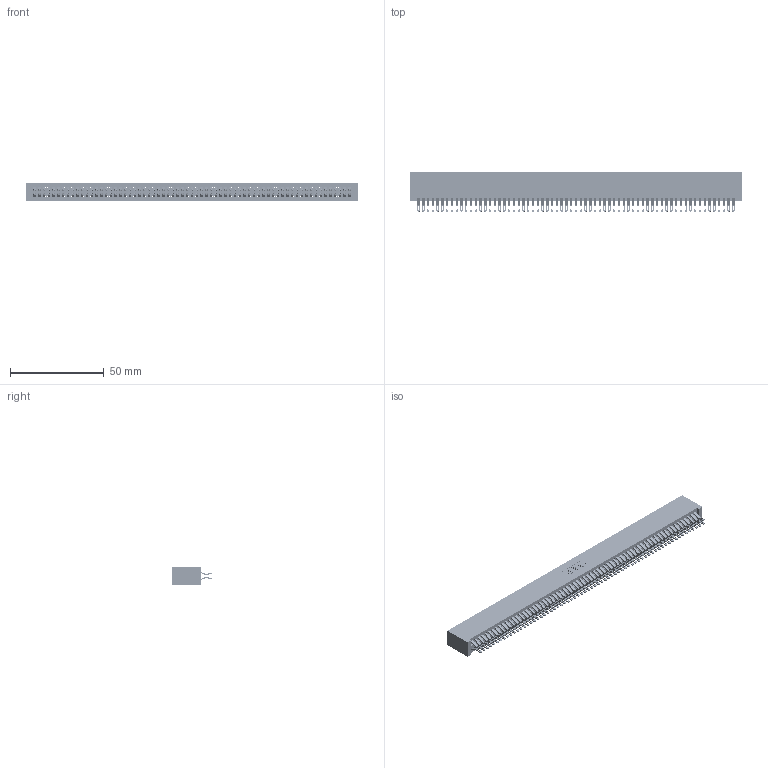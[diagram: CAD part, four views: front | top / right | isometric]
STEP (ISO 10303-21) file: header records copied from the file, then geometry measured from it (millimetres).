
FILE_DESCRIPTION (( 'STEP AP203' ), '1' );
FILE_NAME ('395-134-555-201.STEP', '2018-12-05T04:18:20', ( '' ), ( '' ), 'SwSTEP 2.0', 'SolidWorks 2016', '' );
FILE_SCHEMA (( 'CONFIG_CONTROL_DESIGN' ));
Length unit declared in the file: inch
Products named in the file (3): 345-292-001_555 Tail; 345 Part_No Mounting Lugs; 395-134-555-201
Assembly tree (135 placements, depth 2):
  395-134-555-201
    345 Part_No Mounting Lugs
    345-292-001_555 Tail  x134
Bounding box: 176.78 x 21.13 x 9.4 mm (x, y, z)
Volume: 18409.6 mm3; surface area: 29351.8 mm2
Topology: 135 solids, 135 shells, 7622 faces, 24035 edges, 16022 vertices
Faces by surface type: plane 4230, cylinder 3392
Entity records: 49253 total; most frequent: CARTESIAN_POINT 8266, ORIENTED_EDGE 8170, DIRECTION 7221, EDGE_CURVE 4085, LINE 3673, VECTOR 3673, VERTEX_POINT 2722, AXIS2_PLACEMENT_3D 1774
